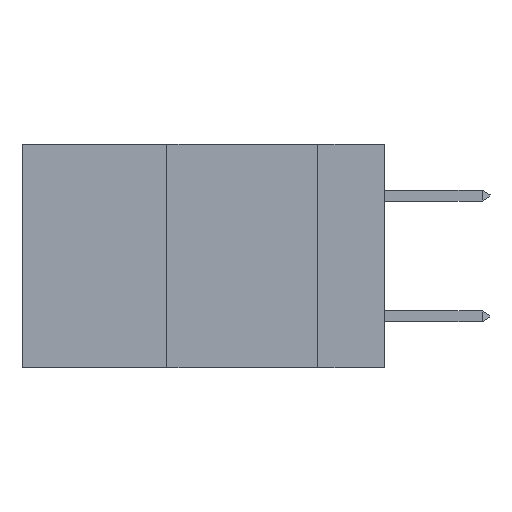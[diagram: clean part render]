
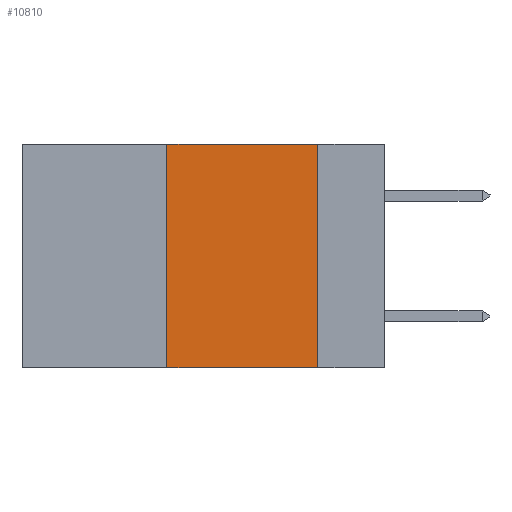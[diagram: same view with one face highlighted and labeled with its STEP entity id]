
A CAD part, left-side view. The second image highlights one B-rep face of the part: STEP entity #10810.
In plain terms, the highlighted planar face has unit normal (-1, 0, 0).
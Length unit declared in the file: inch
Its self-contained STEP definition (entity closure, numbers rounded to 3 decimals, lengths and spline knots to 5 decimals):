
#1283 = EDGE_LOOP ( 'NONE', ( #22036, #29733, #2178, #5679 ) ) ;
#2178 = ORIENTED_EDGE ( 'NONE', *, *, #20909, .F. ) ;
#2905 = LINE ( 'NONE', #13664, #12326 ) ;
#2951 = VECTOR ( 'NONE', #30438, 39.37008 ) ;
#3278 = VECTOR ( 'NONE', #4814, 39.37008 ) ;
#3458 = PLANE ( 'NONE',  #7515 ) ;
#4814 = DIRECTION ( 'NONE',  ( 0., 0., 1. ) ) ;
#5679 = ORIENTED_EDGE ( 'NONE', *, *, #25758, .T. ) ;
#5741 = EDGE_CURVE ( 'NONE', #14827, #15362, #21676, .T. ) ;
#7515 = AXIS2_PLACEMENT_3D ( 'NONE', #29912, #21684, #19263 ) ;
#10810 = ADVANCED_FACE ( 'NONE', ( #18404 ), #3458, .F. ) ;
#12326 = VECTOR ( 'NONE', #26746, 39.37008 ) ;
#13664 = CARTESIAN_POINT ( 'NONE',  ( 0., 0.11, 0. ) ) ;
#14827 = VERTEX_POINT ( 'NONE', #16791 ) ;
#15362 = VERTEX_POINT ( 'NONE', #32123 ) ;
#15502 = LINE ( 'NONE', #30573, #3278 ) ;
#16344 = VECTOR ( 'NONE', #21537, 39.37008 ) ;
#16791 = CARTESIAN_POINT ( 'NONE',  ( 0., 0.36, 0. ) ) ;
#18153 = VERTEX_POINT ( 'NONE', #32975 ) ;
#18404 = FACE_OUTER_BOUND ( 'NONE', #1283, .T. ) ;
#19263 = DIRECTION ( 'NONE',  ( 0., 0., -1. ) ) ;
#20909 = EDGE_CURVE ( 'NONE', #18153, #14827, #15502, .T. ) ;
#21537 = DIRECTION ( 'NONE',  ( 0., -1., 0. ) ) ;
#21676 = LINE ( 'NONE', #33170, #2951 ) ;
#21684 = DIRECTION ( 'NONE',  ( 1., 0., 0. ) ) ;
#22036 = ORIENTED_EDGE ( 'NONE', *, *, #32291, .F. ) ;
#23597 = VERTEX_POINT ( 'NONE', #29354 ) ;
#24092 = LINE ( 'NONE', #26435, #16344 ) ;
#25758 = EDGE_CURVE ( 'NONE', #18153, #23597, #24092, .T. ) ;
#26435 = CARTESIAN_POINT ( 'NONE',  ( 0., 0.6, -0.37 ) ) ;
#26746 = DIRECTION ( 'NONE',  ( 0., 0., -1. ) ) ;
#29354 = CARTESIAN_POINT ( 'NONE',  ( 0., 0.11, -0.37 ) ) ;
#29733 = ORIENTED_EDGE ( 'NONE', *, *, #5741, .F. ) ;
#29912 = CARTESIAN_POINT ( 'NONE',  ( 0., 0.6, 0. ) ) ;
#30438 = DIRECTION ( 'NONE',  ( 0., -1., 0. ) ) ;
#30573 = CARTESIAN_POINT ( 'NONE',  ( 0., 0.36, 0. ) ) ;
#32123 = CARTESIAN_POINT ( 'NONE',  ( 0., 0.11, 0. ) ) ;
#32291 = EDGE_CURVE ( 'NONE', #15362, #23597, #2905, .T. ) ;
#32975 = CARTESIAN_POINT ( 'NONE',  ( 0., 0.36, -0.37 ) ) ;
#33170 = CARTESIAN_POINT ( 'NONE',  ( 0., 0.6, 0. ) ) ;
